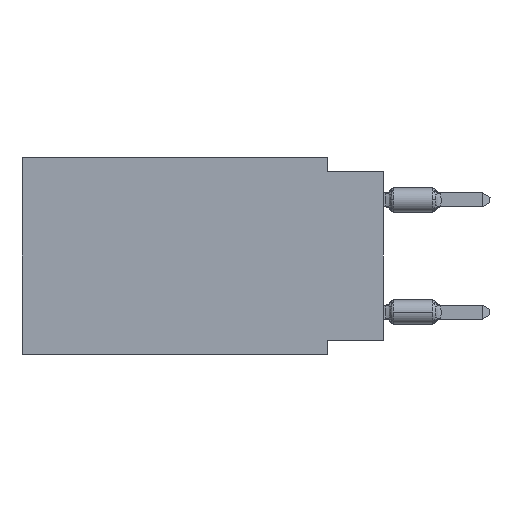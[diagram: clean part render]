
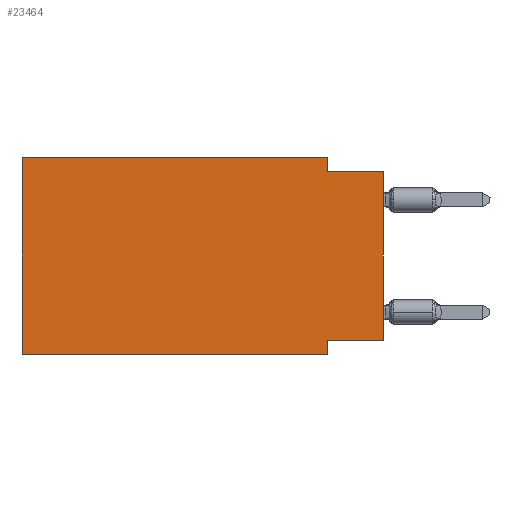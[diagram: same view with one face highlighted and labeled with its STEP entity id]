
A CAD part, left-side view. The second image highlights one B-rep face of the part: STEP entity #23464.
In plain terms, the highlighted planar face has unit normal (-1, 0, 0).
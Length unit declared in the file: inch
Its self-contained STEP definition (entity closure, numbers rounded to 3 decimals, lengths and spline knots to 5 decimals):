
#347 = VECTOR ( 'NONE', #12743, 39.37008 ) ;
#1720 = LINE ( 'NONE', #23287, #18660 ) ;
#2232 = CARTESIAN_POINT ( 'NONE',  ( 0., 0.1, -0.35 ) ) ;
#2602 = AXIS2_PLACEMENT_3D ( 'NONE', #40082, #21890, #25906 ) ;
#4663 = CARTESIAN_POINT ( 'NONE',  ( 0., 0.1, -0.325 ) ) ;
#5008 = ORIENTED_EDGE ( 'NONE', *, *, #22028, .F. ) ;
#5818 = CARTESIAN_POINT ( 'NONE',  ( 0., 0.1, 0. ) ) ;
#5973 = CARTESIAN_POINT ( 'NONE',  ( 0., 0.645, 0. ) ) ;
#7428 = FACE_OUTER_BOUND ( 'NONE', #19865, .T. ) ;
#7778 = EDGE_CURVE ( 'NONE', #28245, #39423, #20028, .T. ) ;
#8703 = LINE ( 'NONE', #5818, #35999 ) ;
#9411 = ORIENTED_EDGE ( 'NONE', *, *, #17301, .F. ) ;
#10244 = ORIENTED_EDGE ( 'NONE', *, *, #7778, .F. ) ;
#10904 = CARTESIAN_POINT ( 'NONE',  ( 0., 0.1, 0. ) ) ;
#11648 = DIRECTION ( 'NONE',  ( 0., -1., 0. ) ) ;
#12743 = DIRECTION ( 'NONE',  ( 0., 0., 1. ) ) ;
#13095 = VECTOR ( 'NONE', #15620, 39.37008 ) ;
#13434 = VECTOR ( 'NONE', #42217, 39.37008 ) ;
#13707 = ORIENTED_EDGE ( 'NONE', *, *, #19057, .F. ) ;
#14857 = ORIENTED_EDGE ( 'NONE', *, *, #25042, .T. ) ;
#15473 = PLANE ( 'NONE',  #2602 ) ;
#15620 = DIRECTION ( 'NONE',  ( 0., 1., 0. ) ) ;
#16751 = LINE ( 'NONE', #30940, #347 ) ;
#17301 = EDGE_CURVE ( 'NONE', #43411, #27888, #18290, .T. ) ;
#18053 = CARTESIAN_POINT ( 'NONE',  ( 0., 0., -0.025 ) ) ;
#18290 = LINE ( 'NONE', #18053, #20798 ) ;
#18660 = VECTOR ( 'NONE', #22827, 39.37008 ) ;
#18962 = CARTESIAN_POINT ( 'NONE',  ( 0., 0., -0.325 ) ) ;
#19057 = EDGE_CURVE ( 'NONE', #37064, #28245, #1720, .T. ) ;
#19188 = LINE ( 'NONE', #18962, #13095 ) ;
#19604 = CARTESIAN_POINT ( 'NONE',  ( 0., 0.645, -0.35 ) ) ;
#19823 = CARTESIAN_POINT ( 'NONE',  ( 0., 0.645, 0. ) ) ;
#19844 = DIRECTION ( 'NONE',  ( 0., 0., -1. ) ) ;
#19865 = EDGE_LOOP ( 'NONE', ( #14857, #9411, #31564, #10244, #13707, #44028, #5008, #21402 ) ) ;
#19872 = CARTESIAN_POINT ( 'NONE',  ( 0., 0.1, -0.025 ) ) ;
#20028 = LINE ( 'NONE', #19823, #21807 ) ;
#20316 = VECTOR ( 'NONE', #41724, 39.37008 ) ;
#20754 = CARTESIAN_POINT ( 'NONE',  ( 0., 0.1, -0.35 ) ) ;
#20798 = VECTOR ( 'NONE', #11648, 39.37008 ) ;
#21202 = CARTESIAN_POINT ( 'NONE',  ( 0., 0., -0.025 ) ) ;
#21402 = ORIENTED_EDGE ( 'NONE', *, *, #39506, .F. ) ;
#21807 = VECTOR ( 'NONE', #29984, 39.37008 ) ;
#21890 = DIRECTION ( 'NONE',  ( 1., 0., 0. ) ) ;
#22028 = EDGE_CURVE ( 'NONE', #42594, #42383, #38439, .T. ) ;
#22827 = DIRECTION ( 'NONE',  ( 0., 0., 1. ) ) ;
#23287 = CARTESIAN_POINT ( 'NONE',  ( 0., 0.645, 0. ) ) ;
#23464 = ADVANCED_FACE ( 'NONE', ( #7428 ), #15473, .F. ) ;
#24762 = VERTEX_POINT ( 'NONE', #28849 ) ;
#25042 = EDGE_CURVE ( 'NONE', #24762, #27888, #16751, .T. ) ;
#25906 = DIRECTION ( 'NONE',  ( 0., 0., -1. ) ) ;
#26849 = CARTESIAN_POINT ( 'NONE',  ( 0., 0.645, -0.35 ) ) ;
#26975 = EDGE_CURVE ( 'NONE', #39423, #43411, #8703, .T. ) ;
#27888 = VERTEX_POINT ( 'NONE', #21202 ) ;
#28245 = VERTEX_POINT ( 'NONE', #5973 ) ;
#28849 = CARTESIAN_POINT ( 'NONE',  ( 0., 0., -0.325 ) ) ;
#29330 = EDGE_CURVE ( 'NONE', #37064, #42383, #45286, .T. ) ;
#29984 = DIRECTION ( 'NONE',  ( 0., -1., 0. ) ) ;
#30940 = CARTESIAN_POINT ( 'NONE',  ( 0., 0., 0. ) ) ;
#31564 = ORIENTED_EDGE ( 'NONE', *, *, #26975, .F. ) ;
#35999 = VECTOR ( 'NONE', #19844, 39.37008 ) ;
#37064 = VERTEX_POINT ( 'NONE', #19604 ) ;
#38439 = LINE ( 'NONE', #2232, #13434 ) ;
#39423 = VERTEX_POINT ( 'NONE', #10904 ) ;
#39506 = EDGE_CURVE ( 'NONE', #24762, #42594, #19188, .T. ) ;
#40082 = CARTESIAN_POINT ( 'NONE',  ( 0., 0.645, 0. ) ) ;
#41724 = DIRECTION ( 'NONE',  ( 0., -1., 0. ) ) ;
#42217 = DIRECTION ( 'NONE',  ( 0., 0., -1. ) ) ;
#42383 = VERTEX_POINT ( 'NONE', #20754 ) ;
#42594 = VERTEX_POINT ( 'NONE', #4663 ) ;
#43411 = VERTEX_POINT ( 'NONE', #19872 ) ;
#44028 = ORIENTED_EDGE ( 'NONE', *, *, #29330, .T. ) ;
#45286 = LINE ( 'NONE', #26849, #20316 ) ;
